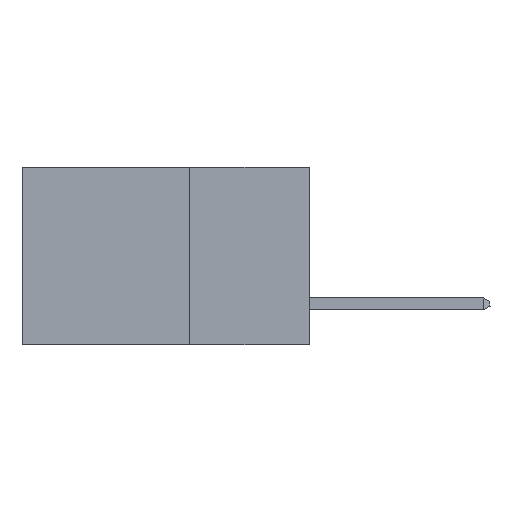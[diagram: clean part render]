
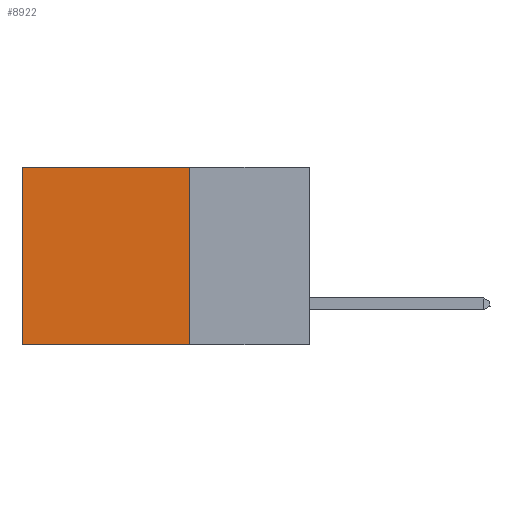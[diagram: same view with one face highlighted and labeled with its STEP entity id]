
A CAD part, left-side view. The second image highlights one B-rep face of the part: STEP entity #8922.
In plain terms, the highlighted planar face has unit normal (-1, 0, 0).
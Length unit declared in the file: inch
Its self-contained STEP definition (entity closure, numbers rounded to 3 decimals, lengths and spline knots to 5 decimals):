
#264 = EDGE_CURVE ( 'NONE', #5405, #4100, #3830, .T. ) ;
#967 = DIRECTION ( 'NONE',  ( 0., 1., 0. ) ) ;
#1247 = PLANE ( 'NONE',  #2825 ) ;
#1787 = VECTOR ( 'NONE', #967, 39.37008 ) ;
#2429 = CARTESIAN_POINT ( 'NONE',  ( 0.2875, 0.25, -0.37 ) ) ;
#2825 = AXIS2_PLACEMENT_3D ( 'NONE', #6762, #2841, #2906 ) ;
#2841 = DIRECTION ( 'NONE',  ( 1., 0., 0. ) ) ;
#2846 = CARTESIAN_POINT ( 'NONE',  ( 0.2875, 0.25, 0. ) ) ;
#2906 = DIRECTION ( 'NONE',  ( 0., 0., -1. ) ) ;
#3150 = ORIENTED_EDGE ( 'NONE', *, *, #5419, .F. ) ;
#3360 = EDGE_LOOP ( 'NONE', ( #5402, #9046, #3150, #9771 ) ) ;
#3361 = VERTEX_POINT ( 'NONE', #6107 ) ;
#3408 = CARTESIAN_POINT ( 'NONE',  ( 0.2875, 0.6, 0. ) ) ;
#3531 = CARTESIAN_POINT ( 'NONE',  ( 0.2875, 0.25, 0. ) ) ;
#3749 = FACE_OUTER_BOUND ( 'NONE', #3360, .T. ) ;
#3830 = LINE ( 'NONE', #6989, #1787 ) ;
#3848 = EDGE_CURVE ( 'NONE', #3361, #8093, #4119, .T. ) ;
#4100 = VERTEX_POINT ( 'NONE', #7160 ) ;
#4119 = LINE ( 'NONE', #2429, #5957 ) ;
#5402 = ORIENTED_EDGE ( 'NONE', *, *, #7164, .T. ) ;
#5405 = VERTEX_POINT ( 'NONE', #3531 ) ;
#5419 = EDGE_CURVE ( 'NONE', #5405, #3361, #9784, .T. ) ;
#5957 = VECTOR ( 'NONE', #10012, 39.37008 ) ;
#6107 = CARTESIAN_POINT ( 'NONE',  ( 0.2875, 0.25, -0.37 ) ) ;
#6762 = CARTESIAN_POINT ( 'NONE',  ( 0.2875, 0.25, 0. ) ) ;
#6898 = CARTESIAN_POINT ( 'NONE',  ( 0.2875, 0.6, -0.37 ) ) ;
#6989 = CARTESIAN_POINT ( 'NONE',  ( 0.2875, 0.25, 0. ) ) ;
#7160 = CARTESIAN_POINT ( 'NONE',  ( 0.2875, 0.6, 0. ) ) ;
#7164 = EDGE_CURVE ( 'NONE', #4100, #8093, #7793, .T. ) ;
#7558 = VECTOR ( 'NONE', #8832, 39.37008 ) ;
#7793 = LINE ( 'NONE', #3408, #7558 ) ;
#8093 = VERTEX_POINT ( 'NONE', #6898 ) ;
#8832 = DIRECTION ( 'NONE',  ( 0., 0., -1. ) ) ;
#8922 = ADVANCED_FACE ( 'NONE', ( #3749 ), #1247, .F. ) ;
#8953 = VECTOR ( 'NONE', #9701, 39.37008 ) ;
#9046 = ORIENTED_EDGE ( 'NONE', *, *, #3848, .F. ) ;
#9701 = DIRECTION ( 'NONE',  ( 0., 0., -1. ) ) ;
#9771 = ORIENTED_EDGE ( 'NONE', *, *, #264, .T. ) ;
#9784 = LINE ( 'NONE', #2846, #8953 ) ;
#10012 = DIRECTION ( 'NONE',  ( 0., 1., 0. ) ) ;
